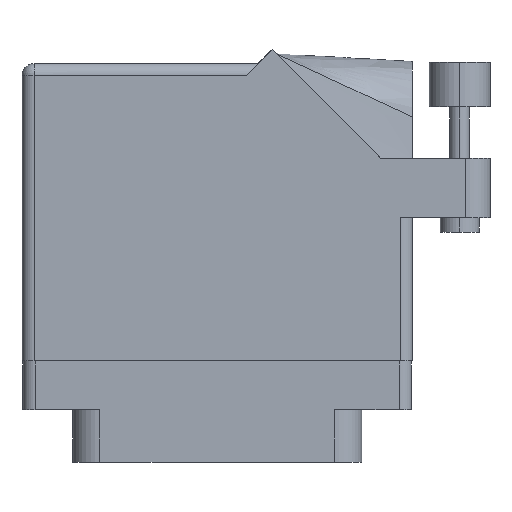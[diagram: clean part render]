
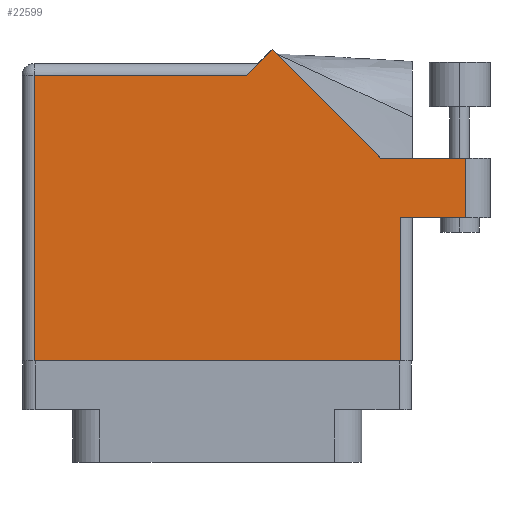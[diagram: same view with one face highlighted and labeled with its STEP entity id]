
A CAD part, front view. The second image highlights one B-rep face of the part: STEP entity #22599.
In plain terms, the highlighted face is planar.
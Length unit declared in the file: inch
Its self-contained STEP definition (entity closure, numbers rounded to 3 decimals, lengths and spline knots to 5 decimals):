
#659 = CARTESIAN_POINT ( 'NONE',  ( 1.28, 0.944, 0.455 ) ) ;
#738 = CARTESIAN_POINT ( 'NONE',  ( 0.28271, 1.50071, 0.455 ) ) ;
#1168 = VERTEX_POINT ( 'NONE', #659 ) ;
#2324 = EDGE_CURVE ( 'NONE', #5638, #1168, #3783, .T. ) ;
#3656 = LINE ( 'NONE', #34497, #19803 ) ;
#3783 = LINE ( 'NONE', #26420, #16846 ) ;
#3936 = LINE ( 'NONE', #20374, #5645 ) ;
#4781 = EDGE_LOOP ( 'NONE', ( #24283, #16045, #12279, #13917, #29747, #18963, #24845, #32293, #28697 ) ) ;
#5015 = CARTESIAN_POINT ( 'NONE',  ( 0.15, 1.368, 0.455 ) ) ;
#5514 = VECTOR ( 'NONE', #24281, 39.37008 ) ;
#5522 = EDGE_CURVE ( 'NONE', #10243, #22665, #21821, .T. ) ;
#5638 = VERTEX_POINT ( 'NONE', #29628 ) ;
#5645 = VECTOR ( 'NONE', #22929, 39.37008 ) ;
#6004 = EDGE_CURVE ( 'NONE', #27177, #15695, #3936, .T. ) ;
#6641 = DIRECTION ( 'NONE',  ( 1., 0., 0. ) ) ;
#6970 = VECTOR ( 'NONE', #35096, 39.37008 ) ;
#7241 = VECTOR ( 'NONE', #15445, 39.37008 ) ;
#7967 = EDGE_CURVE ( 'NONE', #22665, #27177, #18188, .T. ) ;
#8111 = CARTESIAN_POINT ( 'NONE',  ( -1.005, 1.43, 0.455 ) ) ;
#8212 = VECTOR ( 'NONE', #12584, 39.37008 ) ;
#9760 = CARTESIAN_POINT ( 'NONE',  ( 1.405, 0.944, 0.455 ) ) ;
#10243 = VERTEX_POINT ( 'NONE', #5015 ) ;
#10410 = CARTESIAN_POINT ( 'NONE',  ( 0.212, 1.43, 0.455 ) ) ;
#10519 = VERTEX_POINT ( 'NONE', #18752 ) ;
#10718 = EDGE_CURVE ( 'NONE', #15695, #10519, #3656, .T. ) ;
#12158 = CARTESIAN_POINT ( 'NONE',  ( 1.005, 0.637, 0.455 ) ) ;
#12279 = ORIENTED_EDGE ( 'NONE', *, *, #25887, .T. ) ;
#12584 = DIRECTION ( 'NONE',  ( -1., 0., 0. ) ) ;
#12993 = VECTOR ( 'NONE', #19101, 39.37008 ) ;
#13917 = ORIENTED_EDGE ( 'NONE', *, *, #18074, .T. ) ;
#14678 = EDGE_CURVE ( 'NONE', #10519, #5638, #33168, .T. ) ;
#15187 = CARTESIAN_POINT ( 'NONE',  ( -0.943, -0.1, 0.455 ) ) ;
#15445 = DIRECTION ( 'NONE',  ( 0., -1., 0. ) ) ;
#15695 = VERTEX_POINT ( 'NONE', #25025 ) ;
#15785 = CARTESIAN_POINT ( 'NONE',  ( -1.005, 1.368, 0.455 ) ) ;
#16045 = ORIENTED_EDGE ( 'NONE', *, *, #2324, .T. ) ;
#16755 = CARTESIAN_POINT ( 'NONE',  ( 0.83942, 0.944, 0.455 ) ) ;
#16846 = VECTOR ( 'NONE', #20976, 39.37008 ) ;
#18074 = EDGE_CURVE ( 'NONE', #27344, #22092, #30372, .T. ) ;
#18188 = LINE ( 'NONE', #23723, #7241 ) ;
#18456 = EDGE_CURVE ( 'NONE', #22092, #10243, #27322, .T. ) ;
#18752 = CARTESIAN_POINT ( 'NONE',  ( 0.943, 0.637, 0.455 ) ) ;
#18963 = ORIENTED_EDGE ( 'NONE', *, *, #5522, .T. ) ;
#19101 = DIRECTION ( 'NONE',  ( -0.707, 0.707, 0. ) ) ;
#19119 = CARTESIAN_POINT ( 'NONE',  ( -0.943, 1.368, 0.455 ) ) ;
#19359 = DIRECTION ( 'NONE',  ( -1., 0., 0. ) ) ;
#19803 = VECTOR ( 'NONE', #20196, 39.37008 ) ;
#20196 = DIRECTION ( 'NONE',  ( 0., 1., 0. ) ) ;
#20374 = CARTESIAN_POINT ( 'NONE',  ( -1.005, -0.1, 0.455 ) ) ;
#20976 = DIRECTION ( 'NONE',  ( 0., 1., 0. ) ) ;
#21821 = LINE ( 'NONE', #15785, #6970 ) ;
#22092 = VERTEX_POINT ( 'NONE', #738 ) ;
#22599 = ADVANCED_FACE ( 'NONE', ( #32378 ), #33039, .F. ) ;
#22665 = VERTEX_POINT ( 'NONE', #19119 ) ;
#22929 = DIRECTION ( 'NONE',  ( 1., 0., 0. ) ) ;
#23723 = CARTESIAN_POINT ( 'NONE',  ( -0.943, -0.1, 0.455 ) ) ;
#24281 = DIRECTION ( 'NONE',  ( -0.707, -0.707, 0. ) ) ;
#24283 = ORIENTED_EDGE ( 'NONE', *, *, #14678, .T. ) ;
#24845 = ORIENTED_EDGE ( 'NONE', *, *, #7967, .T. ) ;
#25025 = CARTESIAN_POINT ( 'NONE',  ( 0.943, -0.1, 0.455 ) ) ;
#25887 = EDGE_CURVE ( 'NONE', #1168, #27344, #32147, .T. ) ;
#26420 = CARTESIAN_POINT ( 'NONE',  ( 1.28, 0.944, 0.455 ) ) ;
#27177 = VERTEX_POINT ( 'NONE', #15187 ) ;
#27322 = LINE ( 'NONE', #10410, #5514 ) ;
#27344 = VERTEX_POINT ( 'NONE', #16755 ) ;
#28697 = ORIENTED_EDGE ( 'NONE', *, *, #10718, .T. ) ;
#29600 = AXIS2_PLACEMENT_3D ( 'NONE', #8111, #30151, #19359 ) ;
#29628 = CARTESIAN_POINT ( 'NONE',  ( 1.28, 0.637, 0.455 ) ) ;
#29747 = ORIENTED_EDGE ( 'NONE', *, *, #18456, .T. ) ;
#30019 = CARTESIAN_POINT ( 'NONE',  ( 0.83942, 0.944, 0.455 ) ) ;
#30151 = DIRECTION ( 'NONE',  ( 0., 0., -1. ) ) ;
#30372 = LINE ( 'NONE', #30019, #12993 ) ;
#32147 = LINE ( 'NONE', #9760, #8212 ) ;
#32293 = ORIENTED_EDGE ( 'NONE', *, *, #6004, .T. ) ;
#32378 = FACE_OUTER_BOUND ( 'NONE', #4781, .T. ) ;
#33039 = PLANE ( 'NONE',  #29600 ) ;
#33168 = LINE ( 'NONE', #12158, #34468 ) ;
#34468 = VECTOR ( 'NONE', #6641, 39.37008 ) ;
#34497 = CARTESIAN_POINT ( 'NONE',  ( 0.943, 0.637, 0.455 ) ) ;
#35096 = DIRECTION ( 'NONE',  ( -1., 0., 0. ) ) ;
